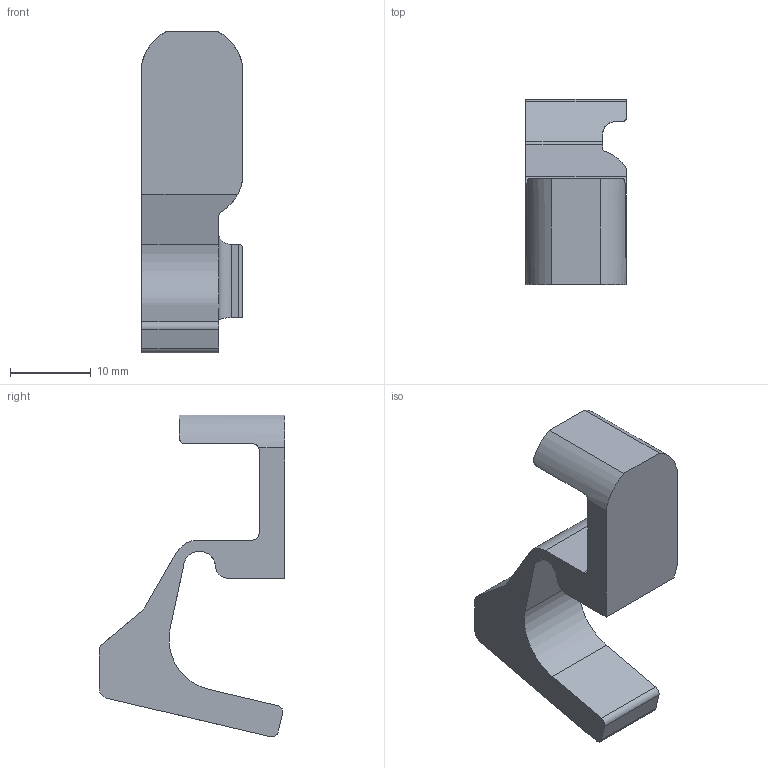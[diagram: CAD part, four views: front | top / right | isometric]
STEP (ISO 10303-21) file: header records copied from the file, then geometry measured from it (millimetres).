
FILE_DESCRIPTION(/* description */ (''),/* implementation_level */ '2;1');
FILE_NAME(/* name */ 'Yankee Boogle Swift Link.stp',/* time_stamp */ '2019-12-25T21:52:25-06:00',/* author */ ('johne'),/* organization */ (''),/* preprocessor_version */ 'ST-DEVELOPER v18',/* originating_system */ 'Autodesk Inventor 2020',/* authorisation */ '');
FILE_SCHEMA (('AUTOMOTIVE_DESIGN { 1 0 10303 214 3 1 1 }'));
Length unit declared in the file: metre
Products named in the file (1): Yankee Boogle Swift Link
Bounding box: 12.45 x 22.99 x 39.92 mm (x, y, z)
Volume: 3222.4 mm3; surface area: 2361.4 mm2
Topology: 1 solids, 1 shells, 38 faces, 108 edges, 72 vertices
Faces by surface type: plane 19, cylinder 19
Entity records: 1332 total; most frequent: CARTESIAN_POINT 264, ORIENTED_EDGE 216, DIRECTION 216, EDGE_CURVE 108, AXIS2_PLACEMENT_3D 74, VERTEX_POINT 72, LINE 68, VECTOR 68
